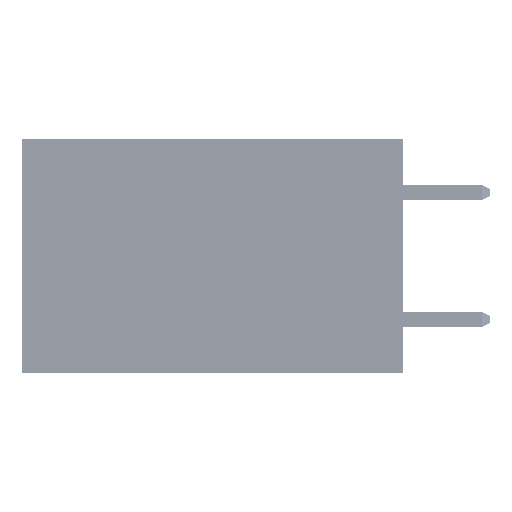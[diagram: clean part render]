
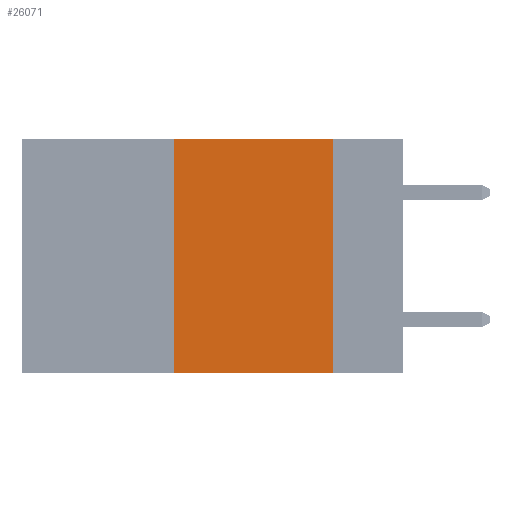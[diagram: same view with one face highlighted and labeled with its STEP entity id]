
A CAD part, left-side view. The second image highlights one B-rep face of the part: STEP entity #26071.
In plain terms, the highlighted planar face has unit normal (-1, 0, 0).
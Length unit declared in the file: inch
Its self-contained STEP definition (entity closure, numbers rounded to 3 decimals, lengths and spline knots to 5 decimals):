
#1801 = DIRECTION ( 'NONE',  ( 0., 0., 1. ) ) ;
#2910 = EDGE_CURVE ( 'NONE', #27849, #46323, #31570, .T. ) ;
#3396 = CARTESIAN_POINT ( 'NONE',  ( 0., 0.6, 0. ) ) ;
#7331 = VECTOR ( 'NONE', #43992, 39.37008 ) ;
#8065 = EDGE_CURVE ( 'NONE', #19032, #46323, #10596, .T. ) ;
#8130 = CARTESIAN_POINT ( 'NONE',  ( 0., 0.11, 0. ) ) ;
#9243 = ORIENTED_EDGE ( 'NONE', *, *, #8065, .F. ) ;
#10404 = EDGE_LOOP ( 'NONE', ( #9243, #12529, #43919, #15847 ) ) ;
#10596 = LINE ( 'NONE', #8130, #19100 ) ;
#12237 = VECTOR ( 'NONE', #1801, 39.37008 ) ;
#12529 = ORIENTED_EDGE ( 'NONE', *, *, #38064, .F. ) ;
#15303 = CARTESIAN_POINT ( 'NONE',  ( 0., 0.11, -0.37 ) ) ;
#15847 = ORIENTED_EDGE ( 'NONE', *, *, #2910, .T. ) ;
#16100 = DIRECTION ( 'NONE',  ( 0., 0., -1. ) ) ;
#16308 = AXIS2_PLACEMENT_3D ( 'NONE', #3396, #30451, #50019 ) ;
#17350 = EDGE_CURVE ( 'NONE', #27849, #36729, #37008, .T. ) ;
#18821 = LINE ( 'NONE', #47554, #7331 ) ;
#19032 = VERTEX_POINT ( 'NONE', #44996 ) ;
#19100 = VECTOR ( 'NONE', #16100, 39.37008 ) ;
#19465 = CARTESIAN_POINT ( 'NONE',  ( 0., 0.6, -0.37 ) ) ;
#21052 = CARTESIAN_POINT ( 'NONE',  ( 0., 0.36, 0. ) ) ;
#21054 = CARTESIAN_POINT ( 'NONE',  ( 0., 0.36, -0.37 ) ) ;
#21442 = CARTESIAN_POINT ( 'NONE',  ( 0., 0.36, 0. ) ) ;
#23064 = VECTOR ( 'NONE', #39225, 39.37008 ) ;
#26071 = ADVANCED_FACE ( 'NONE', ( #29523 ), #49685, .F. ) ;
#27849 = VERTEX_POINT ( 'NONE', #21054 ) ;
#29523 = FACE_OUTER_BOUND ( 'NONE', #10404, .T. ) ;
#30451 = DIRECTION ( 'NONE',  ( 1., 0., 0. ) ) ;
#31570 = LINE ( 'NONE', #19465, #23064 ) ;
#36729 = VERTEX_POINT ( 'NONE', #21442 ) ;
#37008 = LINE ( 'NONE', #21052, #12237 ) ;
#38064 = EDGE_CURVE ( 'NONE', #36729, #19032, #18821, .T. ) ;
#39225 = DIRECTION ( 'NONE',  ( 0., -1., 0. ) ) ;
#43919 = ORIENTED_EDGE ( 'NONE', *, *, #17350, .F. ) ;
#43992 = DIRECTION ( 'NONE',  ( 0., -1., 0. ) ) ;
#44996 = CARTESIAN_POINT ( 'NONE',  ( 0., 0.11, 0. ) ) ;
#46323 = VERTEX_POINT ( 'NONE', #15303 ) ;
#47554 = CARTESIAN_POINT ( 'NONE',  ( 0., 0.6, 0. ) ) ;
#49685 = PLANE ( 'NONE',  #16308 ) ;
#50019 = DIRECTION ( 'NONE',  ( 0., 0., -1. ) ) ;
